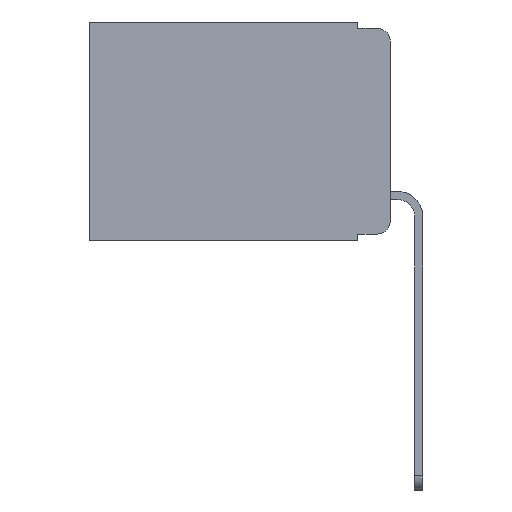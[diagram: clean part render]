
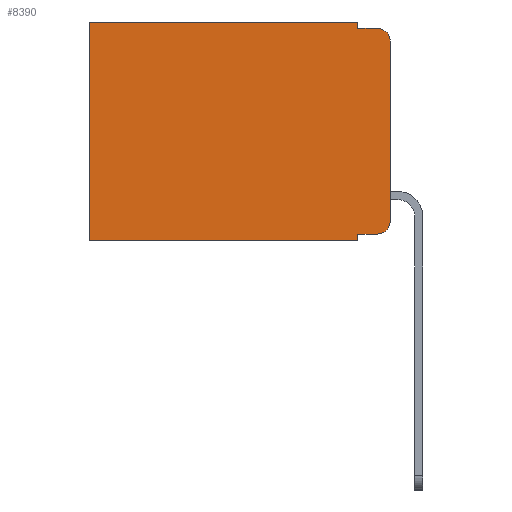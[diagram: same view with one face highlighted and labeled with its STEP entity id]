
A CAD part, left-side view. The second image highlights one B-rep face of the part: STEP entity #8390.
In plain terms, the highlighted planar face has unit normal (-1, 0, 0).
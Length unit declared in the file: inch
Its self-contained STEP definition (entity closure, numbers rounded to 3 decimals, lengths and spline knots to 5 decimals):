
#33 = LINE ( 'NONE', #908, #38 ) ;
#38 = VECTOR ( 'NONE', #3636, 39.37008 ) ;
#253 = CARTESIAN_POINT ( 'NONE',  ( 0.298, 0.02, -0.01 ) ) ;
#420 = CARTESIAN_POINT ( 'NONE',  ( 0.298, 0.051, -0.333 ) ) ;
#670 = VERTEX_POINT ( 'NONE', #8610 ) ;
#794 = ORIENTED_EDGE ( 'NONE', *, *, #4665, .T. ) ;
#823 = VECTOR ( 'NONE', #1780, 39.37008 ) ;
#908 = CARTESIAN_POINT ( 'NONE',  ( 0.298, 0.051, 0. ) ) ;
#1063 = CARTESIAN_POINT ( 'NONE',  ( 0.298, 0.051, -0.333 ) ) ;
#1084 = ORIENTED_EDGE ( 'NONE', *, *, #4519, .T. ) ;
#1160 = DIRECTION ( 'NONE',  ( 0., 0., -1. ) ) ;
#1266 = DIRECTION ( 'NONE',  ( 1., 0., 0. ) ) ;
#1310 = VECTOR ( 'NONE', #1533, 39.37008 ) ;
#1406 = VERTEX_POINT ( 'NONE', #420 ) ;
#1435 = CARTESIAN_POINT ( 'NONE',  ( 0.298, 0.051, -0.01 ) ) ;
#1485 = CARTESIAN_POINT ( 'NONE',  ( 0.298, 0., -0.313 ) ) ;
#1533 = DIRECTION ( 'NONE',  ( 0., 0., -1. ) ) ;
#1548 = AXIS2_PLACEMENT_3D ( 'NONE', #5656, #7501, #11235 ) ;
#1780 = DIRECTION ( 'NONE',  ( 0., 0., -1. ) ) ;
#1944 = EDGE_CURVE ( 'NONE', #1406, #11323, #3710, .T. ) ;
#1948 = LINE ( 'NONE', #6585, #2677 ) ;
#2271 = ORIENTED_EDGE ( 'NONE', *, *, #2552, .F. ) ;
#2303 = DIRECTION ( 'NONE',  ( 0., 0., -1. ) ) ;
#2504 = AXIS2_PLACEMENT_3D ( 'NONE', #11314, #3245, #2303 ) ;
#2552 = EDGE_CURVE ( 'NONE', #9598, #7802, #6863, .T. ) ;
#2559 = EDGE_LOOP ( 'NONE', ( #9546, #794, #2271, #7047, #7079, #6110, #8429, #8915, #1084, #5687 ) ) ;
#2677 = VECTOR ( 'NONE', #10913, 39.37008 ) ;
#3047 = CARTESIAN_POINT ( 'NONE',  ( 0.298, 0.051, 0. ) ) ;
#3095 = DIRECTION ( 'NONE',  ( 0., -1., 0. ) ) ;
#3237 = CIRCLE ( 'NONE', #2504, 0.02 ) ;
#3245 = DIRECTION ( 'NONE',  ( -1., 0., 0. ) ) ;
#3293 = PLANE ( 'NONE',  #5408 ) ;
#3636 = DIRECTION ( 'NONE',  ( 0., 0., -1. ) ) ;
#3710 = LINE ( 'NONE', #10954, #5974 ) ;
#4112 = CARTESIAN_POINT ( 'NONE',  ( 0.298, 0.473, 0. ) ) ;
#4192 = LINE ( 'NONE', #5272, #1310 ) ;
#4519 = EDGE_CURVE ( 'NONE', #1406, #7521, #4680, .T. ) ;
#4539 = EDGE_CURVE ( 'NONE', #11323, #4632, #1948, .T. ) ;
#4632 = VERTEX_POINT ( 'NONE', #10067 ) ;
#4665 = EDGE_CURVE ( 'NONE', #670, #7802, #3237, .T. ) ;
#4680 = LINE ( 'NONE', #1063, #5518 ) ;
#4696 = LINE ( 'NONE', #10027, #5711 ) ;
#4854 = EDGE_CURVE ( 'NONE', #670, #7635, #6255, .T. ) ;
#5046 = CARTESIAN_POINT ( 'NONE',  ( 0.298, 0.02, -0.333 ) ) ;
#5272 = CARTESIAN_POINT ( 'NONE',  ( 0.298, 0.473, 0. ) ) ;
#5383 = EDGE_CURVE ( 'NONE', #10075, #9612, #4696, .T. ) ;
#5408 = AXIS2_PLACEMENT_3D ( 'NONE', #11359, #1266, #8573 ) ;
#5518 = VECTOR ( 'NONE', #7357, 39.37008 ) ;
#5586 = DIRECTION ( 'NONE',  ( 0., 1., 0. ) ) ;
#5656 = CARTESIAN_POINT ( 'NONE',  ( 0.298, 0.02, -0.313 ) ) ;
#5658 = CARTESIAN_POINT ( 'NONE',  ( 0.298, 0.051, -0.01 ) ) ;
#5687 = ORIENTED_EDGE ( 'NONE', *, *, #11494, .T. ) ;
#5711 = VECTOR ( 'NONE', #5586, 39.37008 ) ;
#5974 = VECTOR ( 'NONE', #1160, 39.37008 ) ;
#6110 = ORIENTED_EDGE ( 'NONE', *, *, #9872, .T. ) ;
#6255 = LINE ( 'NONE', #9837, #823 ) ;
#6585 = CARTESIAN_POINT ( 'NONE',  ( 0.298, 0., -0.343 ) ) ;
#6634 = FACE_OUTER_BOUND ( 'NONE', #2559, .T. ) ;
#6863 = LINE ( 'NONE', #1435, #8042 ) ;
#7047 = ORIENTED_EDGE ( 'NONE', *, *, #10840, .F. ) ;
#7079 = ORIENTED_EDGE ( 'NONE', *, *, #5383, .T. ) ;
#7357 = DIRECTION ( 'NONE',  ( 0., -1., 0. ) ) ;
#7501 = DIRECTION ( 'NONE',  ( -1., 0., 0. ) ) ;
#7521 = VERTEX_POINT ( 'NONE', #5046 ) ;
#7635 = VERTEX_POINT ( 'NONE', #1485 ) ;
#7802 = VERTEX_POINT ( 'NONE', #253 ) ;
#8042 = VECTOR ( 'NONE', #3095, 39.37008 ) ;
#8390 = ADVANCED_FACE ( 'NONE', ( #6634 ), #3293, .F. ) ;
#8429 = ORIENTED_EDGE ( 'NONE', *, *, #4539, .F. ) ;
#8573 = DIRECTION ( 'NONE',  ( 0., 0., -1. ) ) ;
#8610 = CARTESIAN_POINT ( 'NONE',  ( 0.298, 0., -0.03 ) ) ;
#8687 = CIRCLE ( 'NONE', #1548, 0.02 ) ;
#8915 = ORIENTED_EDGE ( 'NONE', *, *, #1944, .F. ) ;
#9063 = CARTESIAN_POINT ( 'NONE',  ( 0.298, 0.051, -0.343 ) ) ;
#9546 = ORIENTED_EDGE ( 'NONE', *, *, #4854, .F. ) ;
#9598 = VERTEX_POINT ( 'NONE', #5658 ) ;
#9612 = VERTEX_POINT ( 'NONE', #4112 ) ;
#9837 = CARTESIAN_POINT ( 'NONE',  ( 0.298, 0., 0. ) ) ;
#9872 = EDGE_CURVE ( 'NONE', #9612, #4632, #4192, .T. ) ;
#10027 = CARTESIAN_POINT ( 'NONE',  ( 0.298, 0., 0. ) ) ;
#10067 = CARTESIAN_POINT ( 'NONE',  ( 0.298, 0.473, -0.343 ) ) ;
#10075 = VERTEX_POINT ( 'NONE', #3047 ) ;
#10840 = EDGE_CURVE ( 'NONE', #10075, #9598, #33, .T. ) ;
#10913 = DIRECTION ( 'NONE',  ( 0., 1., 0. ) ) ;
#10954 = CARTESIAN_POINT ( 'NONE',  ( 0.298, 0.051, 0. ) ) ;
#11235 = DIRECTION ( 'NONE',  ( 0., 0., -1. ) ) ;
#11314 = CARTESIAN_POINT ( 'NONE',  ( 0.298, 0.02, -0.03 ) ) ;
#11323 = VERTEX_POINT ( 'NONE', #9063 ) ;
#11359 = CARTESIAN_POINT ( 'NONE',  ( 0.298, 0., 0. ) ) ;
#11494 = EDGE_CURVE ( 'NONE', #7521, #7635, #8687, .T. ) ;
